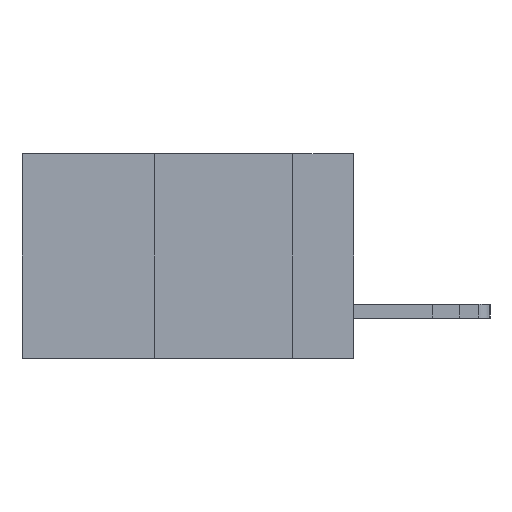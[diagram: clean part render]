
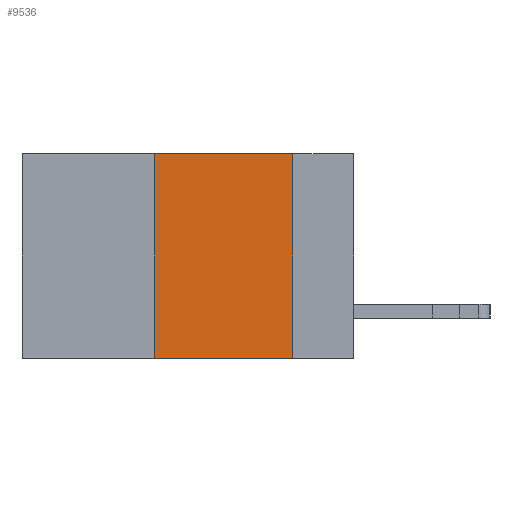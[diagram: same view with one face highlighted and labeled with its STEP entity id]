
A CAD part, left-side view. The second image highlights one B-rep face of the part: STEP entity #9536.
In plain terms, the highlighted planar face has unit normal (-1, 0, 0).
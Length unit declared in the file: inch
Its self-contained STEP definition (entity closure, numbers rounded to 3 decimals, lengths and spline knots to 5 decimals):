
#392 = VERTEX_POINT ( 'NONE', #5106 ) ;
#549 = VERTEX_POINT ( 'NONE', #2113 ) ;
#1586 = FACE_OUTER_BOUND ( 'NONE', #5496, .T. ) ;
#2113 = CARTESIAN_POINT ( 'NONE',  ( 0., 0.11, 0. ) ) ;
#2123 = CARTESIAN_POINT ( 'NONE',  ( 0., 0.6, -0.37 ) ) ;
#2326 = LINE ( 'NONE', #7324, #4342 ) ;
#2527 = EDGE_CURVE ( 'NONE', #549, #8746, #2326, .T. ) ;
#2595 = ORIENTED_EDGE ( 'NONE', *, *, #9590, .T. ) ;
#2662 = DIRECTION ( 'NONE',  ( 0., 0., -1. ) ) ;
#3251 = EDGE_CURVE ( 'NONE', #392, #3649, #16129, .T. ) ;
#3649 = VERTEX_POINT ( 'NONE', #12356 ) ;
#4342 = VECTOR ( 'NONE', #5842, 39.37008 ) ;
#4875 = DIRECTION ( 'NONE',  ( 0., 0., 1. ) ) ;
#5106 = CARTESIAN_POINT ( 'NONE',  ( 0., 0.36, -0.37 ) ) ;
#5496 = EDGE_LOOP ( 'NONE', ( #15043, #6163, #7483, #2595 ) ) ;
#5842 = DIRECTION ( 'NONE',  ( 0., 0., -1. ) ) ;
#6163 = ORIENTED_EDGE ( 'NONE', *, *, #7125, .F. ) ;
#6493 = VECTOR ( 'NONE', #13291, 39.37008 ) ;
#6607 = DIRECTION ( 'NONE',  ( 1., 0., 0. ) ) ;
#7125 = EDGE_CURVE ( 'NONE', #3649, #549, #14500, .T. ) ;
#7324 = CARTESIAN_POINT ( 'NONE',  ( 0., 0.11, 0. ) ) ;
#7483 = ORIENTED_EDGE ( 'NONE', *, *, #3251, .F. ) ;
#8567 = AXIS2_PLACEMENT_3D ( 'NONE', #13977, #6607, #2662 ) ;
#8746 = VERTEX_POINT ( 'NONE', #10604 ) ;
#9536 = ADVANCED_FACE ( 'NONE', ( #1586 ), #10148, .F. ) ;
#9590 = EDGE_CURVE ( 'NONE', #392, #8746, #14696, .T. ) ;
#10148 = PLANE ( 'NONE',  #8567 ) ;
#10604 = CARTESIAN_POINT ( 'NONE',  ( 0., 0.11, -0.37 ) ) ;
#12192 = VECTOR ( 'NONE', #4875, 39.37008 ) ;
#12356 = CARTESIAN_POINT ( 'NONE',  ( 0., 0.36, 0. ) ) ;
#13148 = CARTESIAN_POINT ( 'NONE',  ( 0., 0.6, 0. ) ) ;
#13291 = DIRECTION ( 'NONE',  ( 0., -1., 0. ) ) ;
#13977 = CARTESIAN_POINT ( 'NONE',  ( 0., 0.6, 0. ) ) ;
#14288 = DIRECTION ( 'NONE',  ( 0., -1., 0. ) ) ;
#14500 = LINE ( 'NONE', #13148, #6493 ) ;
#14656 = CARTESIAN_POINT ( 'NONE',  ( 0., 0.36, 0. ) ) ;
#14696 = LINE ( 'NONE', #2123, #14883 ) ;
#14883 = VECTOR ( 'NONE', #14288, 39.37008 ) ;
#15043 = ORIENTED_EDGE ( 'NONE', *, *, #2527, .F. ) ;
#16129 = LINE ( 'NONE', #14656, #12192 ) ;
